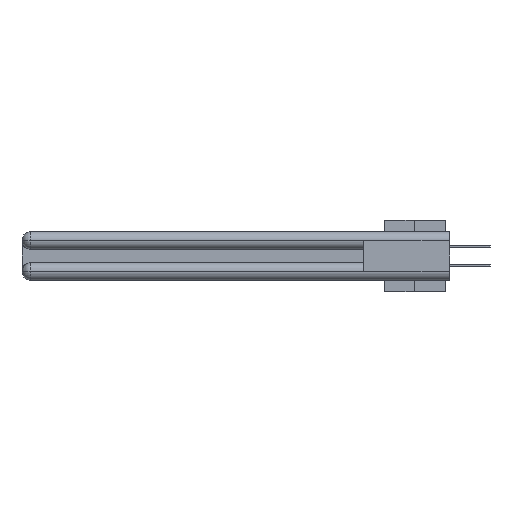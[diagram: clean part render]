
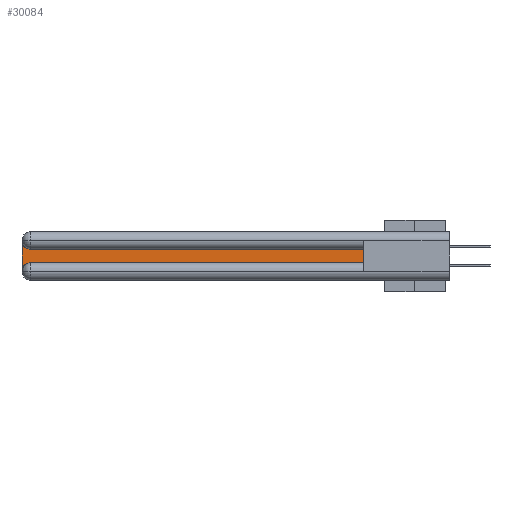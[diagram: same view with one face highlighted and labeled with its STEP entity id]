
A CAD part, left-side view. The second image highlights one B-rep face of the part: STEP entity #30084.
In plain terms, the highlighted planar face has unit normal (-1, 0, 0).
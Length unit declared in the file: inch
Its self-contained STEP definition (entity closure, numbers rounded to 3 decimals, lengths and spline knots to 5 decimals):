
#649 = DIRECTION ( 'NONE',  ( 1., 0., 0. ) ) ;
#800 = CARTESIAN_POINT ( 'NONE',  ( 0.075, 3., -0.1225 ) ) ;
#2731 = CARTESIAN_POINT ( 'NONE',  ( 0.075, 3., -0.2175 ) ) ;
#6498 = VERTEX_POINT ( 'NONE', #39820 ) ;
#9278 = VERTEX_POINT ( 'NONE', #34615 ) ;
#9507 = FACE_OUTER_BOUND ( 'NONE', #13208, .T. ) ;
#10358 = VERTEX_POINT ( 'NONE', #36980 ) ;
#10435 = CARTESIAN_POINT ( 'NONE',  ( 0.075, 0.6, -0.1225 ) ) ;
#11404 = EDGE_CURVE ( 'NONE', #9278, #30728, #39684, .T. ) ;
#12042 = ORIENTED_EDGE ( 'NONE', *, *, #31958, .T. ) ;
#12899 = DIRECTION ( 'NONE',  ( 0., 0., -1. ) ) ;
#13208 = EDGE_LOOP ( 'NONE', ( #12042, #41536, #27583, #39766, #46213, #32705 ) ) ;
#15508 = LINE ( 'NONE', #10435, #26075 ) ;
#16084 = VECTOR ( 'NONE', #32294, 39.37008 ) ;
#17582 = DIRECTION ( 'NONE',  ( 0., 1., 0. ) ) ;
#18940 = DIRECTION ( 'NONE',  ( 0., 0., -1. ) ) ;
#20872 = AXIS2_PLACEMENT_3D ( 'NONE', #25675, #36752, #32847 ) ;
#21805 = CIRCLE ( 'NONE', #20872, 0.06 ) ;
#23096 = DIRECTION ( 'NONE',  ( 0., 0., 1. ) ) ;
#24140 = AXIS2_PLACEMENT_3D ( 'NONE', #800, #649, #18940 ) ;
#24740 = EDGE_CURVE ( 'NONE', #10358, #9278, #32026, .T. ) ;
#25282 = CARTESIAN_POINT ( 'NONE',  ( 0.075, 0.6, -0.2175 ) ) ;
#25558 = LINE ( 'NONE', #25282, #16084 ) ;
#25675 = CARTESIAN_POINT ( 'NONE',  ( 0.075, 2.94, -0.2775 ) ) ;
#26075 = VECTOR ( 'NONE', #17582, 39.37008 ) ;
#26251 = VECTOR ( 'NONE', #12899, 39.37008 ) ;
#27156 = DIRECTION ( 'NONE',  ( 0., 0., -1. ) ) ;
#27316 = VECTOR ( 'NONE', #23096, 39.37008 ) ;
#27583 = ORIENTED_EDGE ( 'NONE', *, *, #11404, .T. ) ;
#29684 = CARTESIAN_POINT ( 'NONE',  ( 0.075, 0.6, -0.2175 ) ) ;
#30084 = ADVANCED_FACE ( 'NONE', ( #9507 ), #32638, .F. ) ;
#30728 = VERTEX_POINT ( 'NONE', #43386 ) ;
#31958 = EDGE_CURVE ( 'NONE', #34592, #10358, #15508, .T. ) ;
#32026 = CIRCLE ( 'NONE', #37518, 0.06 ) ;
#32079 = VERTEX_POINT ( 'NONE', #29684 ) ;
#32294 = DIRECTION ( 'NONE',  ( 0., -1., 0. ) ) ;
#32638 = PLANE ( 'NONE',  #24140 ) ;
#32705 = ORIENTED_EDGE ( 'NONE', *, *, #42397, .T. ) ;
#32847 = DIRECTION ( 'NONE',  ( 0., 0., -1. ) ) ;
#34031 = CARTESIAN_POINT ( 'NONE',  ( 0.075, 2.94, -0.0625 ) ) ;
#34592 = VERTEX_POINT ( 'NONE', #34784 ) ;
#34615 = CARTESIAN_POINT ( 'NONE',  ( 0.075, 3., -0.0625 ) ) ;
#34784 = CARTESIAN_POINT ( 'NONE',  ( 0.075, 0.6, -0.1225 ) ) ;
#36752 = DIRECTION ( 'NONE',  ( 1., 0., 0. ) ) ;
#36799 = LINE ( 'NONE', #44475, #27316 ) ;
#36980 = CARTESIAN_POINT ( 'NONE',  ( 0.075, 2.94, -0.1225 ) ) ;
#37518 = AXIS2_PLACEMENT_3D ( 'NONE', #34031, #44765, #27156 ) ;
#39546 = EDGE_CURVE ( 'NONE', #30728, #6498, #21805, .T. ) ;
#39684 = LINE ( 'NONE', #2731, #26251 ) ;
#39766 = ORIENTED_EDGE ( 'NONE', *, *, #39546, .T. ) ;
#39820 = CARTESIAN_POINT ( 'NONE',  ( 0.075, 2.94, -0.2175 ) ) ;
#41536 = ORIENTED_EDGE ( 'NONE', *, *, #24740, .T. ) ;
#42397 = EDGE_CURVE ( 'NONE', #32079, #34592, #36799, .T. ) ;
#43071 = EDGE_CURVE ( 'NONE', #6498, #32079, #25558, .T. ) ;
#43386 = CARTESIAN_POINT ( 'NONE',  ( 0.075, 3., -0.2775 ) ) ;
#44475 = CARTESIAN_POINT ( 'NONE',  ( 0.075, 0.6, -0.2175 ) ) ;
#44765 = DIRECTION ( 'NONE',  ( 1., 0., 0. ) ) ;
#46213 = ORIENTED_EDGE ( 'NONE', *, *, #43071, .T. ) ;
